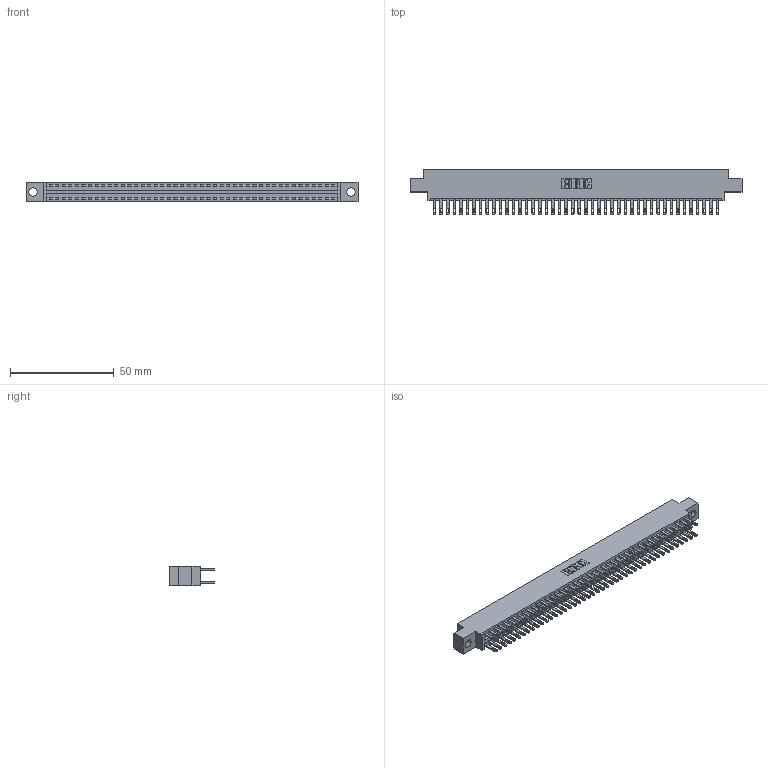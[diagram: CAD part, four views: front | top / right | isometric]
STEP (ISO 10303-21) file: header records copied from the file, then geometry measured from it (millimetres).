
FILE_DESCRIPTION (( 'STEP AP203' ), '1' );
FILE_NAME ('346-088-500-804.STEP', '2018-08-29T23:39:12', ( '' ), ( '' ), 'SwSTEP 2.0', 'SolidWorks 2016', '' );
FILE_SCHEMA (( 'CONFIG_CONTROL_DESIGN' ));
Length unit declared in the file: inch
Products named in the file (3): 345-292-001_345-293-100; 346-088-500-804; 346 Part_0.170 Offset - 0.156 Dia-TH
Assembly tree (89 placements, depth 2):
  346-088-500-804
    346 Part_0.170 Offset - 0.156 Dia-TH
    345-292-001_345-293-100  x88
Bounding box: 160.27 x 21.84 x 9.4 mm (x, y, z)
Volume: 15670.7 mm3; surface area: 22485.9 mm2
Topology: 89 solids, 89 shells, 4350 faces, 13277 edges, 8850 vertices
Faces by surface type: plane 2632, cylinder 1718
Entity records: 28511 total; most frequent: CARTESIAN_POINT 4696, ORIENTED_EDGE 4630, DIRECTION 4191, EDGE_CURVE 2315, LINE 2003, VECTOR 2003, VERTEX_POINT 1542, AXIS2_PLACEMENT_3D 1094
